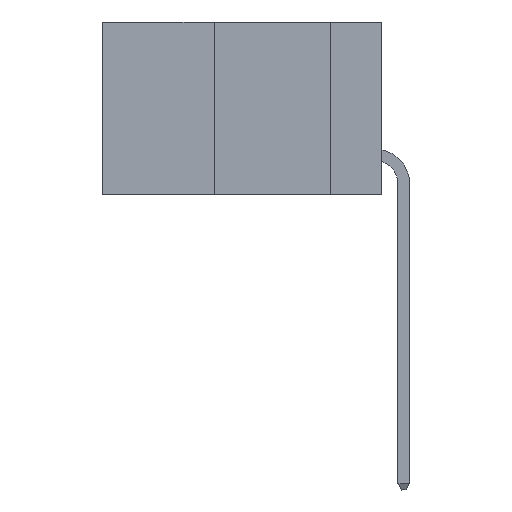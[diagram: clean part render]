
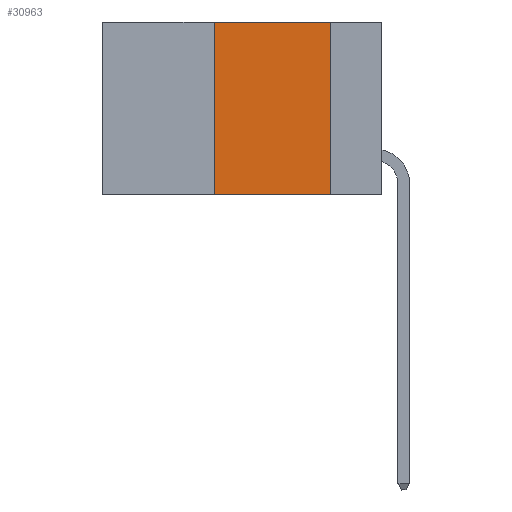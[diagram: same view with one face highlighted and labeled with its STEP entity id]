
A CAD part, left-side view. The second image highlights one B-rep face of the part: STEP entity #30963.
In plain terms, the highlighted planar face has unit normal (-1, 0, 0).
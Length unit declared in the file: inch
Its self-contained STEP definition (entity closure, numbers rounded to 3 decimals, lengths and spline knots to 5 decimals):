
#697 = LINE ( 'NONE', #24817, #7146 ) ;
#932 = EDGE_CURVE ( 'NONE', #25450, #16675, #31054, .T. ) ;
#7146 = VECTOR ( 'NONE', #24979, 39.37008 ) ;
#7657 = EDGE_CURVE ( 'NONE', #31685, #16675, #21756, .T. ) ;
#8296 = EDGE_CURVE ( 'NONE', #37249, #31685, #10179, .T. ) ;
#9480 = EDGE_CURVE ( 'NONE', #25450, #37249, #697, .T. ) ;
#10179 = LINE ( 'NONE', #18852, #36582 ) ;
#14977 = EDGE_LOOP ( 'NONE', ( #16898, #47262, #25204, #15929 ) ) ;
#15929 = ORIENTED_EDGE ( 'NONE', *, *, #932, .T. ) ;
#16675 = VERTEX_POINT ( 'NONE', #46136 ) ;
#16898 = ORIENTED_EDGE ( 'NONE', *, *, #7657, .F. ) ;
#17904 = CARTESIAN_POINT ( 'NONE',  ( 0., 0.36, -0.37 ) ) ;
#18852 = CARTESIAN_POINT ( 'NONE',  ( 0., 0.6, 0. ) ) ;
#21756 = LINE ( 'NONE', #41126, #41621 ) ;
#21931 = PLANE ( 'NONE',  #27023 ) ;
#22300 = DIRECTION ( 'NONE',  ( 0., -1., 0. ) ) ;
#24817 = CARTESIAN_POINT ( 'NONE',  ( 0., 0.36, 0. ) ) ;
#24979 = DIRECTION ( 'NONE',  ( 0., 0., 1. ) ) ;
#25204 = ORIENTED_EDGE ( 'NONE', *, *, #9480, .F. ) ;
#25450 = VERTEX_POINT ( 'NONE', #17904 ) ;
#25716 = DIRECTION ( 'NONE',  ( 0., 0., -1. ) ) ;
#27023 = AXIS2_PLACEMENT_3D ( 'NONE', #36991, #48064, #25716 ) ;
#27226 = CARTESIAN_POINT ( 'NONE',  ( 0., 0.36, 0. ) ) ;
#29913 = CARTESIAN_POINT ( 'NONE',  ( 0., 0.11, 0. ) ) ;
#30963 = ADVANCED_FACE ( 'NONE', ( #38091 ), #21931, .F. ) ;
#31054 = LINE ( 'NONE', #38081, #36314 ) ;
#31685 = VERTEX_POINT ( 'NONE', #29913 ) ;
#33475 = DIRECTION ( 'NONE',  ( 0., 0., -1. ) ) ;
#36314 = VECTOR ( 'NONE', #45594, 39.37008 ) ;
#36582 = VECTOR ( 'NONE', #22300, 39.37008 ) ;
#36991 = CARTESIAN_POINT ( 'NONE',  ( 0., 0.6, 0. ) ) ;
#37249 = VERTEX_POINT ( 'NONE', #27226 ) ;
#38081 = CARTESIAN_POINT ( 'NONE',  ( 0., 0.6, -0.37 ) ) ;
#38091 = FACE_OUTER_BOUND ( 'NONE', #14977, .T. ) ;
#41126 = CARTESIAN_POINT ( 'NONE',  ( 0., 0.11, 0. ) ) ;
#41621 = VECTOR ( 'NONE', #33475, 39.37008 ) ;
#45594 = DIRECTION ( 'NONE',  ( 0., -1., 0. ) ) ;
#46136 = CARTESIAN_POINT ( 'NONE',  ( 0., 0.11, -0.37 ) ) ;
#47262 = ORIENTED_EDGE ( 'NONE', *, *, #8296, .F. ) ;
#48064 = DIRECTION ( 'NONE',  ( 1., 0., 0. ) ) ;
